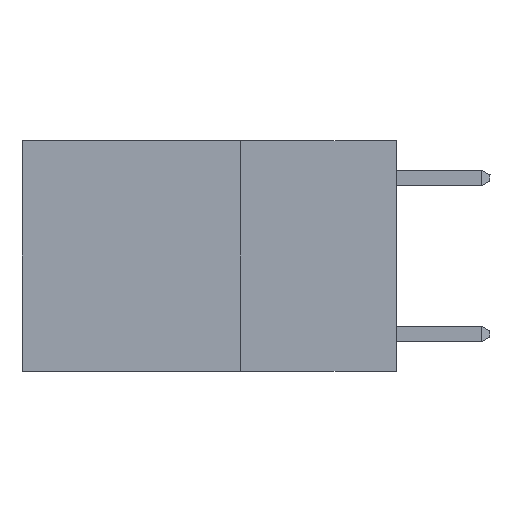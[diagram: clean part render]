
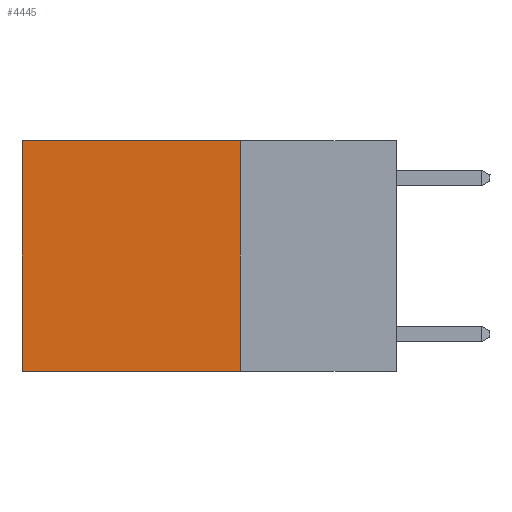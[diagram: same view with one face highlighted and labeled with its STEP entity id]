
A CAD part, left-side view. The second image highlights one B-rep face of the part: STEP entity #4445.
In plain terms, the highlighted planar face has unit normal (-1, 0, 0).
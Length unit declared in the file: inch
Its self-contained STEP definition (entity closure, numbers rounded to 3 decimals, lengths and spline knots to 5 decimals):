
#241 = EDGE_CURVE ( 'NONE', #8378, #11430, #16110, .T. ) ;
#407 = DIRECTION ( 'NONE',  ( 0., 1., 0. ) ) ;
#2284 = VECTOR ( 'NONE', #407, 39.37008 ) ;
#2462 = VERTEX_POINT ( 'NONE', #4473 ) ;
#2736 = FACE_OUTER_BOUND ( 'NONE', #11176, .T. ) ;
#3242 = CARTESIAN_POINT ( 'NONE',  ( 0.2625, 0.25, 0. ) ) ;
#4191 = CARTESIAN_POINT ( 'NONE',  ( 0.2625, 0.6, 0. ) ) ;
#4445 = ADVANCED_FACE ( 'NONE', ( #2736 ), #13062, .F. ) ;
#4457 = AXIS2_PLACEMENT_3D ( 'NONE', #19482, #9417, #16236 ) ;
#4473 = CARTESIAN_POINT ( 'NONE',  ( 0.2625, 0.6, 0. ) ) ;
#5037 = ORIENTED_EDGE ( 'NONE', *, *, #19901, .T. ) ;
#5137 = EDGE_CURVE ( 'NONE', #11430, #5541, #8226, .T. ) ;
#5541 = VERTEX_POINT ( 'NONE', #7182 ) ;
#7182 = CARTESIAN_POINT ( 'NONE',  ( 0.2625, 0.6, -0.37 ) ) ;
#7504 = VECTOR ( 'NONE', #16398, 39.37008 ) ;
#8213 = ORIENTED_EDGE ( 'NONE', *, *, #5137, .F. ) ;
#8226 = LINE ( 'NONE', #14970, #7504 ) ;
#8378 = VERTEX_POINT ( 'NONE', #3242 ) ;
#9224 = LINE ( 'NONE', #4191, #15709 ) ;
#9417 = DIRECTION ( 'NONE',  ( 1., 0., 0. ) ) ;
#9937 = ORIENTED_EDGE ( 'NONE', *, *, #241, .F. ) ;
#11176 = EDGE_LOOP ( 'NONE', ( #12929, #8213, #9937, #5037 ) ) ;
#11430 = VERTEX_POINT ( 'NONE', #16104 ) ;
#12929 = ORIENTED_EDGE ( 'NONE', *, *, #20897, .T. ) ;
#13062 = PLANE ( 'NONE',  #4457 ) ;
#14005 = CARTESIAN_POINT ( 'NONE',  ( 0.2625, 0.25, 0. ) ) ;
#14463 = CARTESIAN_POINT ( 'NONE',  ( 0.2625, 0.25, 0. ) ) ;
#14970 = CARTESIAN_POINT ( 'NONE',  ( 0.2625, 0.25, -0.37 ) ) ;
#15659 = LINE ( 'NONE', #14005, #2284 ) ;
#15709 = VECTOR ( 'NONE', #15713, 39.37008 ) ;
#15713 = DIRECTION ( 'NONE',  ( 0., 0., -1. ) ) ;
#16104 = CARTESIAN_POINT ( 'NONE',  ( 0.2625, 0.25, -0.37 ) ) ;
#16110 = LINE ( 'NONE', #14463, #16628 ) ;
#16236 = DIRECTION ( 'NONE',  ( 0., 0., -1. ) ) ;
#16398 = DIRECTION ( 'NONE',  ( 0., 1., 0. ) ) ;
#16628 = VECTOR ( 'NONE', #21125, 39.37008 ) ;
#19482 = CARTESIAN_POINT ( 'NONE',  ( 0.2625, 0.25, 0. ) ) ;
#19901 = EDGE_CURVE ( 'NONE', #8378, #2462, #15659, .T. ) ;
#20897 = EDGE_CURVE ( 'NONE', #2462, #5541, #9224, .T. ) ;
#21125 = DIRECTION ( 'NONE',  ( 0., 0., -1. ) ) ;
